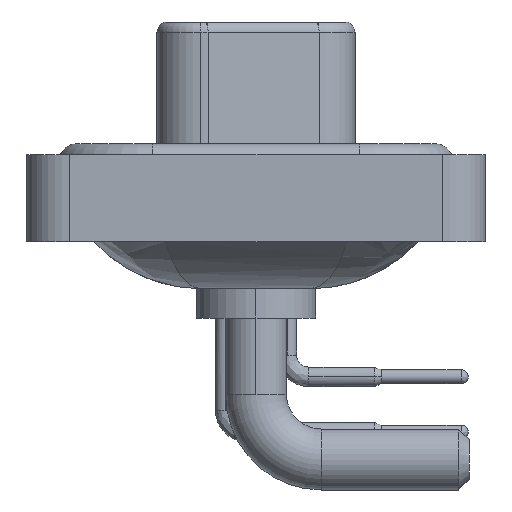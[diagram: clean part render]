
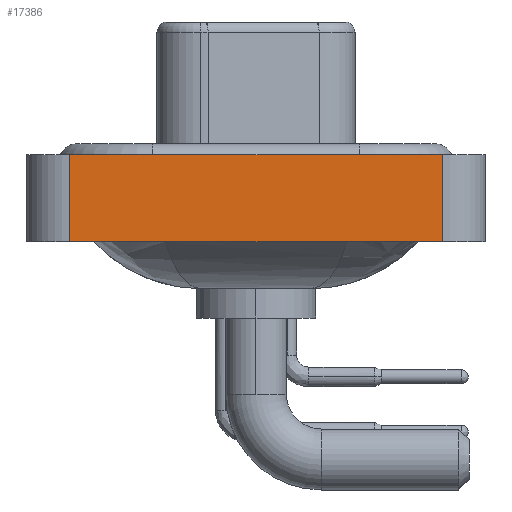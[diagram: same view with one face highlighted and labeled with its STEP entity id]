
A CAD part, left-side view. The second image highlights one B-rep face of the part: STEP entity #17386.
In plain terms, the highlighted planar face has unit normal (-1, 0, 0).
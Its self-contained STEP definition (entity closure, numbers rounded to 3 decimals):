
#1799 = FACE_OUTER_BOUND ( 'NONE', #10060, .T. ) ;
#1958 = CARTESIAN_POINT ( 'NONE',  ( -7.35, -8.55, 0.4 ) ) ;
#3324 = DIRECTION ( 'NONE',  ( 0., -1., 0. ) ) ;
#3527 = EDGE_CURVE ( 'NONE', #5882, #11089, #17309, .T. ) ;
#3876 = CARTESIAN_POINT ( 'NONE',  ( -7.35, 8.55, -3.6 ) ) ;
#4132 = DIRECTION ( 'NONE',  ( 0., 0., 1. ) ) ;
#4962 = CARTESIAN_POINT ( 'NONE',  ( -7.35, 8.55, -3.6 ) ) ;
#5530 = EDGE_CURVE ( 'NONE', #27218, #11089, #10766, .T. ) ;
#5882 = VERTEX_POINT ( 'NONE', #10167 ) ;
#6176 = PLANE ( 'NONE',  #14893 ) ;
#8326 = VERTEX_POINT ( 'NONE', #3876 ) ;
#8967 = DIRECTION ( 'NONE',  ( 0., 0., 1. ) ) ;
#9160 = CARTESIAN_POINT ( 'NONE',  ( -7.35, -8.55, -3.6 ) ) ;
#10060 = EDGE_LOOP ( 'NONE', ( #11529, #23784, #13869, #21891 ) ) ;
#10167 = CARTESIAN_POINT ( 'NONE',  ( -7.35, -8.55, -3.6 ) ) ;
#10336 = DIRECTION ( 'NONE',  ( -1., 0., 0. ) ) ;
#10354 = DIRECTION ( 'NONE',  ( 0., -1., 0. ) ) ;
#10469 = CARTESIAN_POINT ( 'NONE',  ( -7.35, -8.55, -3.6 ) ) ;
#10766 = LINE ( 'NONE', #1958, #20486 ) ;
#11019 = EDGE_CURVE ( 'NONE', #8326, #27218, #13382, .T. ) ;
#11089 = VERTEX_POINT ( 'NONE', #20011 ) ;
#11529 = ORIENTED_EDGE ( 'NONE', *, *, #3527, .T. ) ;
#13382 = LINE ( 'NONE', #4962, #13792 ) ;
#13792 = VECTOR ( 'NONE', #8967, 1000. ) ;
#13869 = ORIENTED_EDGE ( 'NONE', *, *, #11019, .F. ) ;
#14519 = VECTOR ( 'NONE', #23297, 1000. ) ;
#14893 = AXIS2_PLACEMENT_3D ( 'NONE', #10469, #10336, #4132 ) ;
#15325 = VECTOR ( 'NONE', #3324, 1000. ) ;
#15991 = CARTESIAN_POINT ( 'NONE',  ( -7.35, -8.55, -3.6 ) ) ;
#17206 = EDGE_CURVE ( 'NONE', #8326, #5882, #21961, .T. ) ;
#17309 = LINE ( 'NONE', #9160, #14519 ) ;
#17386 = ADVANCED_FACE ( 'NONE', ( #1799 ), #6176, .T. ) ;
#20011 = CARTESIAN_POINT ( 'NONE',  ( -7.35, -8.55, 0.4 ) ) ;
#20486 = VECTOR ( 'NONE', #10354, 1000. ) ;
#21891 = ORIENTED_EDGE ( 'NONE', *, *, #17206, .T. ) ;
#21961 = LINE ( 'NONE', #15991, #15325 ) ;
#23297 = DIRECTION ( 'NONE',  ( 0., 0., 1. ) ) ;
#23784 = ORIENTED_EDGE ( 'NONE', *, *, #5530, .F. ) ;
#24439 = CARTESIAN_POINT ( 'NONE',  ( -7.35, 8.55, 0.4 ) ) ;
#27218 = VERTEX_POINT ( 'NONE', #24439 ) ;
